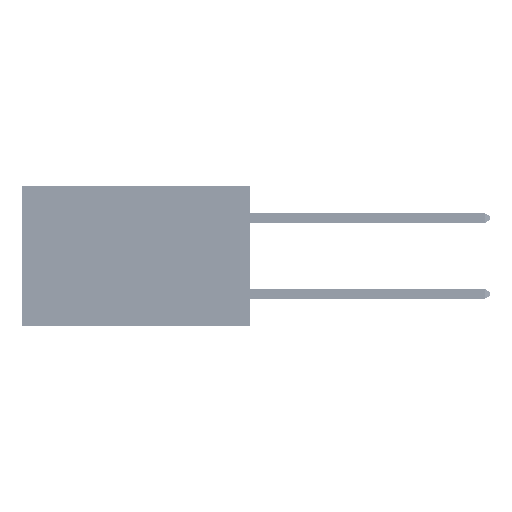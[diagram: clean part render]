
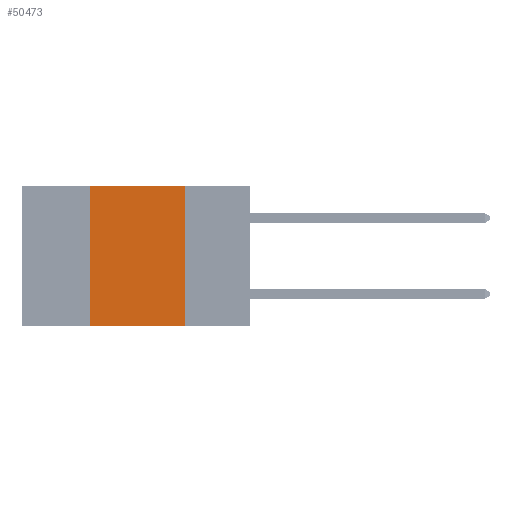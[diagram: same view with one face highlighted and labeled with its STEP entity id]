
A CAD part, left-side view. The second image highlights one B-rep face of the part: STEP entity #50473.
In plain terms, the highlighted planar face has unit normal (-1, 0, 0).
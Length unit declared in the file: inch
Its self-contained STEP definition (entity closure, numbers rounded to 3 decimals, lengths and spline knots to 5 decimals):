
#5904 = CARTESIAN_POINT ( 'NONE',  ( 0., 0.6, 0. ) ) ;
#7656 = CARTESIAN_POINT ( 'NONE',  ( 0., 0.6, -0.37 ) ) ;
#8127 = CARTESIAN_POINT ( 'NONE',  ( 0., 0.42, 0. ) ) ;
#9983 = LINE ( 'NONE', #30175, #25165 ) ;
#10311 = EDGE_CURVE ( 'NONE', #29897, #34956, #9983, .T. ) ;
#10633 = ORIENTED_EDGE ( 'NONE', *, *, #10311, .F. ) ;
#11314 = DIRECTION ( 'NONE',  ( 0., 0., -1. ) ) ;
#12448 = DIRECTION ( 'NONE',  ( 0., 0., 1. ) ) ;
#14585 = VECTOR ( 'NONE', #39935, 39.37008 ) ;
#16914 = VERTEX_POINT ( 'NONE', #39418 ) ;
#19665 = PLANE ( 'NONE',  #36841 ) ;
#20807 = LINE ( 'NONE', #8127, #27495 ) ;
#23952 = VERTEX_POINT ( 'NONE', #50104 ) ;
#24169 = VECTOR ( 'NONE', #42986, 39.37008 ) ;
#25165 = VECTOR ( 'NONE', #29911, 39.37008 ) ;
#26800 = CARTESIAN_POINT ( 'NONE',  ( 0., 0.17, -0.37 ) ) ;
#27495 = VECTOR ( 'NONE', #12448, 39.37008 ) ;
#29897 = VERTEX_POINT ( 'NONE', #47927 ) ;
#29911 = DIRECTION ( 'NONE',  ( 0., 0., -1. ) ) ;
#30175 = CARTESIAN_POINT ( 'NONE',  ( 0., 0.17, 0. ) ) ;
#31892 = LINE ( 'NONE', #7656, #14585 ) ;
#32013 = ORIENTED_EDGE ( 'NONE', *, *, #35119, .T. ) ;
#34956 = VERTEX_POINT ( 'NONE', #26800 ) ;
#35119 = EDGE_CURVE ( 'NONE', #16914, #34956, #31892, .T. ) ;
#35161 = LINE ( 'NONE', #5904, #24169 ) ;
#36544 = CARTESIAN_POINT ( 'NONE',  ( 0., 0.6, 0. ) ) ;
#36841 = AXIS2_PLACEMENT_3D ( 'NONE', #36544, #44646, #11314 ) ;
#37118 = EDGE_LOOP ( 'NONE', ( #10633, #49650, #39743, #32013 ) ) ;
#37358 = EDGE_CURVE ( 'NONE', #23952, #29897, #35161, .T. ) ;
#39418 = CARTESIAN_POINT ( 'NONE',  ( 0., 0.42, -0.37 ) ) ;
#39743 = ORIENTED_EDGE ( 'NONE', *, *, #52628, .F. ) ;
#39935 = DIRECTION ( 'NONE',  ( 0., -1., 0. ) ) ;
#42986 = DIRECTION ( 'NONE',  ( 0., -1., 0. ) ) ;
#44646 = DIRECTION ( 'NONE',  ( 1., 0., 0. ) ) ;
#47927 = CARTESIAN_POINT ( 'NONE',  ( 0., 0.17, 0. ) ) ;
#48126 = FACE_OUTER_BOUND ( 'NONE', #37118, .T. ) ;
#49650 = ORIENTED_EDGE ( 'NONE', *, *, #37358, .F. ) ;
#50104 = CARTESIAN_POINT ( 'NONE',  ( 0., 0.42, 0. ) ) ;
#50473 = ADVANCED_FACE ( 'NONE', ( #48126 ), #19665, .F. ) ;
#52628 = EDGE_CURVE ( 'NONE', #16914, #23952, #20807, .T. ) ;
